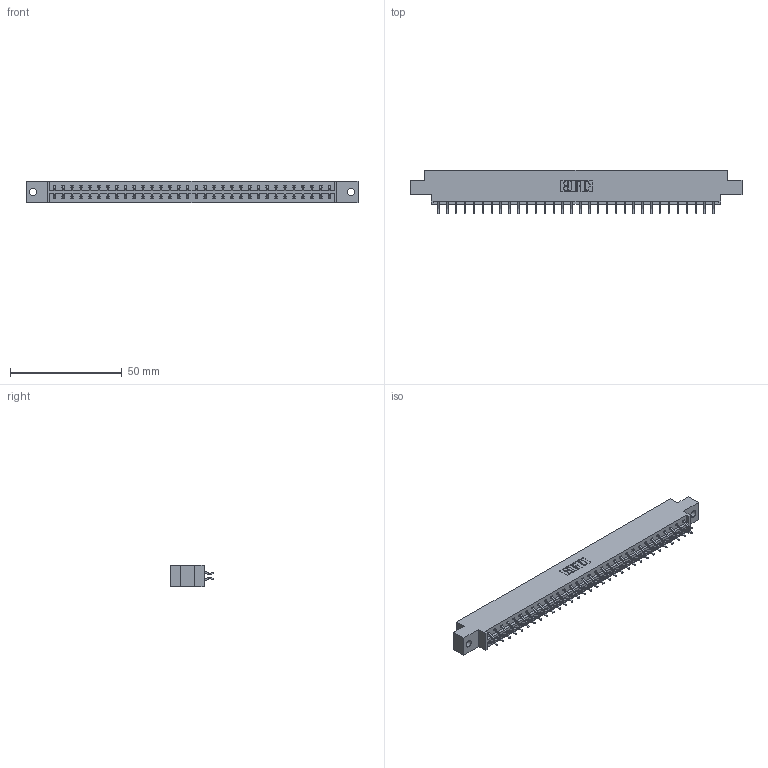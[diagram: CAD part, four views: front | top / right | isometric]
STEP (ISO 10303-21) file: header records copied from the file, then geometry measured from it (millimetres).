
FILE_DESCRIPTION (( 'STEP AP203' ), '1' );
FILE_NAME ('833-064-556-802.STEP', '2020-06-05T07:48:09', ( '' ), ( '' ), 'SwSTEP 2.0', 'SolidWorks 2020', '' );
FILE_SCHEMA (( 'CONFIG_CONTROL_DESIGN' ));
Length unit declared in the file: inch
Products named in the file (3): 345-292-001_556 Tail; 833-064-556-802; 833 Part_Offset - .128 Dia
Assembly tree (65 placements, depth 2):
  833-064-556-802
    833 Part_Offset - .128 Dia
    345-292-001_556 Tail  x64
Bounding box: 148.34 x 19.57 x 9.4 mm (x, y, z)
Volume: 14783.7 mm3; surface area: 17255 mm2
Topology: 65 solids, 65 shells, 3830 faces, 11395 edges, 7510 vertices
Faces by surface type: plane 2634, cylinder 1196
Entity records: 22235 total; most frequent: CARTESIAN_POINT 3714, ORIENTED_EDGE 3638, DIRECTION 3179, EDGE_CURVE 1819, LINE 1683, VECTOR 1683, VERTEX_POINT 1210, AXIS2_PLACEMENT_3D 748
